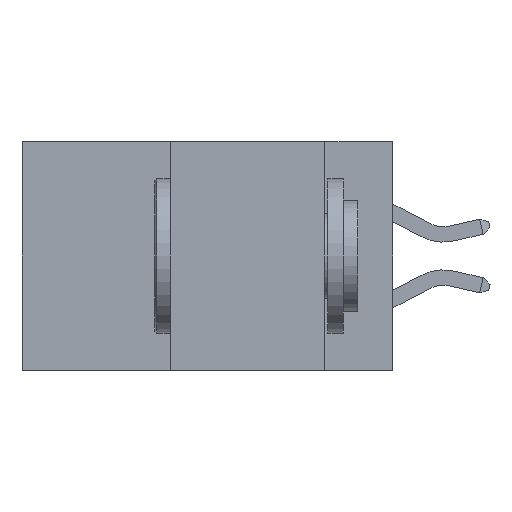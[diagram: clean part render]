
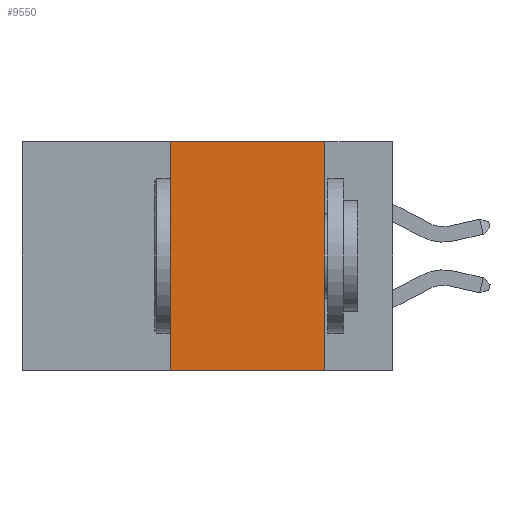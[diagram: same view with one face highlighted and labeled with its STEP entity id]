
A CAD part, left-side view. The second image highlights one B-rep face of the part: STEP entity #9550.
In plain terms, the highlighted planar face has unit normal (-1, 0, 0).
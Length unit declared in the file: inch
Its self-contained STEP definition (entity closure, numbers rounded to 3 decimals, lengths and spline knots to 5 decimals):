
#381 = DIRECTION ( 'NONE',  ( 0., -1., 0. ) ) ;
#493 = DIRECTION ( 'NONE',  ( 0., -1., 0. ) ) ;
#523 = LINE ( 'NONE', #8071, #2124 ) ;
#883 = LINE ( 'NONE', #10231, #9792 ) ;
#885 = CARTESIAN_POINT ( 'NONE',  ( 0., 0.11, 0. ) ) ;
#1095 = DIRECTION ( 'NONE',  ( 1., 0., 0. ) ) ;
#1203 = CARTESIAN_POINT ( 'NONE',  ( 0., 0.11, 0. ) ) ;
#1207 = VERTEX_POINT ( 'NONE', #3442 ) ;
#1324 = ORIENTED_EDGE ( 'NONE', *, *, #7937, .T. ) ;
#1692 = VERTEX_POINT ( 'NONE', #10568 ) ;
#1770 = DIRECTION ( 'NONE',  ( 0., 0., 1. ) ) ;
#2124 = VECTOR ( 'NONE', #381, 39.37008 ) ;
#2484 = EDGE_LOOP ( 'NONE', ( #7379, #3352, #9058, #1324 ) ) ;
#2645 = DIRECTION ( 'NONE',  ( 0., 0., -1. ) ) ;
#2954 = EDGE_CURVE ( 'NONE', #1692, #1207, #883, .T. ) ;
#3352 = ORIENTED_EDGE ( 'NONE', *, *, #8029, .F. ) ;
#3442 = CARTESIAN_POINT ( 'NONE',  ( 0., 0.36, 0. ) ) ;
#3725 = EDGE_CURVE ( 'NONE', #9529, #4680, #4378, .T. ) ;
#4021 = LINE ( 'NONE', #10843, #7771 ) ;
#4378 = LINE ( 'NONE', #885, #8270 ) ;
#4680 = VERTEX_POINT ( 'NONE', #5417 ) ;
#5417 = CARTESIAN_POINT ( 'NONE',  ( 0., 0.11, -0.37 ) ) ;
#5876 = FACE_OUTER_BOUND ( 'NONE', #2484, .T. ) ;
#6221 = PLANE ( 'NONE',  #6427 ) ;
#6427 = AXIS2_PLACEMENT_3D ( 'NONE', #7916, #1095, #7105 ) ;
#7105 = DIRECTION ( 'NONE',  ( 0., 0., -1. ) ) ;
#7379 = ORIENTED_EDGE ( 'NONE', *, *, #3725, .F. ) ;
#7771 = VECTOR ( 'NONE', #493, 39.37008 ) ;
#7916 = CARTESIAN_POINT ( 'NONE',  ( 0., 0.6, 0. ) ) ;
#7937 = EDGE_CURVE ( 'NONE', #1692, #4680, #523, .T. ) ;
#8029 = EDGE_CURVE ( 'NONE', #1207, #9529, #4021, .T. ) ;
#8071 = CARTESIAN_POINT ( 'NONE',  ( 0., 0.6, -0.37 ) ) ;
#8270 = VECTOR ( 'NONE', #2645, 39.37008 ) ;
#9058 = ORIENTED_EDGE ( 'NONE', *, *, #2954, .F. ) ;
#9529 = VERTEX_POINT ( 'NONE', #1203 ) ;
#9550 = ADVANCED_FACE ( 'NONE', ( #5876 ), #6221, .F. ) ;
#9792 = VECTOR ( 'NONE', #1770, 39.37008 ) ;
#10231 = CARTESIAN_POINT ( 'NONE',  ( 0., 0.36, 0. ) ) ;
#10568 = CARTESIAN_POINT ( 'NONE',  ( 0., 0.36, -0.37 ) ) ;
#10843 = CARTESIAN_POINT ( 'NONE',  ( 0., 0.6, 0. ) ) ;
